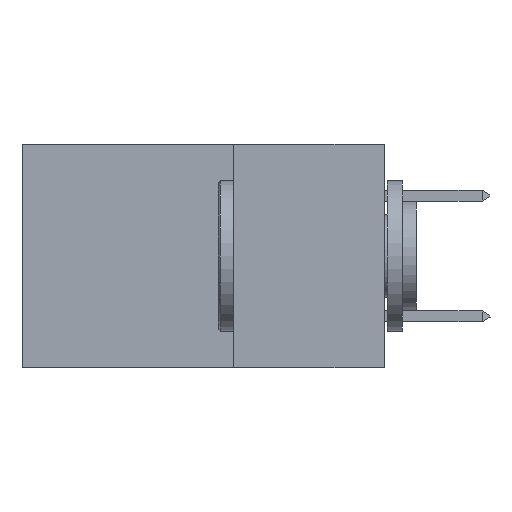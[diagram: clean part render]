
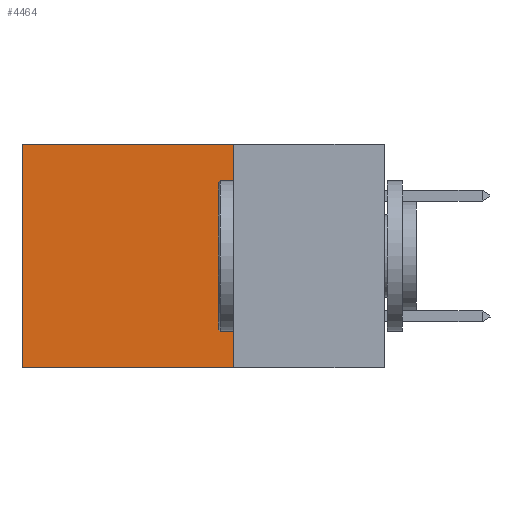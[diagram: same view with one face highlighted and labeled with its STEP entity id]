
A CAD part, left-side view. The second image highlights one B-rep face of the part: STEP entity #4464.
In plain terms, the highlighted planar face has unit normal (-1, 0, 0).
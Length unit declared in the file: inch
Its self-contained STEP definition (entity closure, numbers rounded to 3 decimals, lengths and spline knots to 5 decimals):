
#112 = LINE ( 'NONE', #4879, #15488 ) ;
#1231 = PLANE ( 'NONE',  #35901 ) ;
#2841 = VERTEX_POINT ( 'NONE', #28125 ) ;
#4464 = ADVANCED_FACE ( 'NONE', ( #6165 ), #1231, .F. ) ;
#4879 = CARTESIAN_POINT ( 'NONE',  ( 0.2875, 0.25, -0.37 ) ) ;
#5266 = CARTESIAN_POINT ( 'NONE',  ( 0.2875, 0.25, 0. ) ) ;
#6165 = FACE_OUTER_BOUND ( 'NONE', #17836, .T. ) ;
#7029 = EDGE_CURVE ( 'NONE', #18022, #16077, #17867, .T. ) ;
#8220 = EDGE_CURVE ( 'NONE', #16077, #30786, #112, .T. ) ;
#9576 = DIRECTION ( 'NONE',  ( 0., 1., 0. ) ) ;
#10997 = VECTOR ( 'NONE', #9576, 39.37008 ) ;
#11281 = DIRECTION ( 'NONE',  ( 1., 0., 0. ) ) ;
#12988 = ORIENTED_EDGE ( 'NONE', *, *, #8220, .F. ) ;
#13434 = DIRECTION ( 'NONE',  ( 0., 0., -1. ) ) ;
#14289 = ORIENTED_EDGE ( 'NONE', *, *, #19463, .T. ) ;
#14397 = ORIENTED_EDGE ( 'NONE', *, *, #21188, .T. ) ;
#15488 = VECTOR ( 'NONE', #38550, 39.37008 ) ;
#16077 = VERTEX_POINT ( 'NONE', #34916 ) ;
#17836 = EDGE_LOOP ( 'NONE', ( #14289, #12988, #31093, #14397 ) ) ;
#17867 = LINE ( 'NONE', #5266, #23138 ) ;
#18022 = VERTEX_POINT ( 'NONE', #39022 ) ;
#18535 = DIRECTION ( 'NONE',  ( 0., 0., -1. ) ) ;
#19107 = LINE ( 'NONE', #27845, #10997 ) ;
#19463 = EDGE_CURVE ( 'NONE', #2841, #30786, #33580, .T. ) ;
#20103 = DIRECTION ( 'NONE',  ( 0., 0., -1. ) ) ;
#21188 = EDGE_CURVE ( 'NONE', #18022, #2841, #19107, .T. ) ;
#23054 = CARTESIAN_POINT ( 'NONE',  ( 0.2875, 0.25, 0. ) ) ;
#23138 = VECTOR ( 'NONE', #13434, 39.37008 ) ;
#25499 = VECTOR ( 'NONE', #18535, 39.37008 ) ;
#27845 = CARTESIAN_POINT ( 'NONE',  ( 0.2875, 0.25, 0. ) ) ;
#27884 = CARTESIAN_POINT ( 'NONE',  ( 0.2875, 0.6, 0. ) ) ;
#28125 = CARTESIAN_POINT ( 'NONE',  ( 0.2875, 0.6, 0. ) ) ;
#30044 = CARTESIAN_POINT ( 'NONE',  ( 0.2875, 0.6, -0.37 ) ) ;
#30786 = VERTEX_POINT ( 'NONE', #30044 ) ;
#31093 = ORIENTED_EDGE ( 'NONE', *, *, #7029, .F. ) ;
#33580 = LINE ( 'NONE', #27884, #25499 ) ;
#34916 = CARTESIAN_POINT ( 'NONE',  ( 0.2875, 0.25, -0.37 ) ) ;
#35901 = AXIS2_PLACEMENT_3D ( 'NONE', #23054, #11281, #20103 ) ;
#38550 = DIRECTION ( 'NONE',  ( 0., 1., 0. ) ) ;
#39022 = CARTESIAN_POINT ( 'NONE',  ( 0.2875, 0.25, 0. ) ) ;
